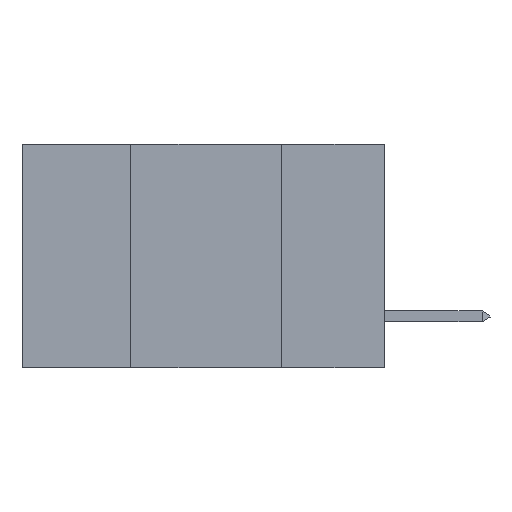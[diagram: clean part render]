
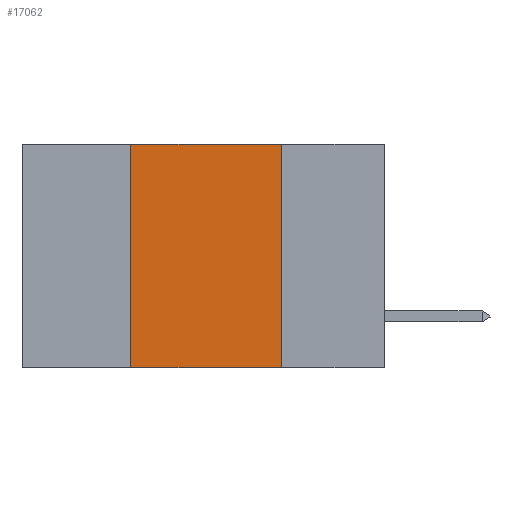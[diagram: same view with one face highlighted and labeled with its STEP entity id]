
A CAD part, left-side view. The second image highlights one B-rep face of the part: STEP entity #17062.
In plain terms, the highlighted planar face has unit normal (-1, 0, 0).
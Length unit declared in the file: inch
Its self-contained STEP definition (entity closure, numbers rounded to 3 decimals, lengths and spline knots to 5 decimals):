
#70 = VECTOR ( 'NONE', #6772, 39.37008 ) ;
#285 = FACE_OUTER_BOUND ( 'NONE', #20038, .T. ) ;
#735 = CARTESIAN_POINT ( 'NONE',  ( 0., 0.6, 0. ) ) ;
#895 = VERTEX_POINT ( 'NONE', #28042 ) ;
#1100 = CARTESIAN_POINT ( 'NONE',  ( 0., 0.17, -0.37 ) ) ;
#2730 = ORIENTED_EDGE ( 'NONE', *, *, #9376, .T. ) ;
#2997 = DIRECTION ( 'NONE',  ( 0., 0., -1. ) ) ;
#4866 = AXIS2_PLACEMENT_3D ( 'NONE', #735, #16094, #2997 ) ;
#5042 = EDGE_CURVE ( 'NONE', #6911, #27293, #19323, .T. ) ;
#5829 = LINE ( 'NONE', #23668, #70 ) ;
#6772 = DIRECTION ( 'NONE',  ( 0., 0., -1. ) ) ;
#6911 = VERTEX_POINT ( 'NONE', #19561 ) ;
#7093 = PLANE ( 'NONE',  #4866 ) ;
#7493 = LINE ( 'NONE', #16509, #17658 ) ;
#7668 = ORIENTED_EDGE ( 'NONE', *, *, #7778, .F. ) ;
#7778 = EDGE_CURVE ( 'NONE', #27293, #895, #23218, .T. ) ;
#8568 = VERTEX_POINT ( 'NONE', #1100 ) ;
#8936 = EDGE_CURVE ( 'NONE', #895, #8568, #5829, .T. ) ;
#9376 = EDGE_CURVE ( 'NONE', #6911, #8568, #7493, .T. ) ;
#14802 = CARTESIAN_POINT ( 'NONE',  ( 0., 0.6, 0. ) ) ;
#16094 = DIRECTION ( 'NONE',  ( 1., 0., 0. ) ) ;
#16509 = CARTESIAN_POINT ( 'NONE',  ( 0., 0.6, -0.37 ) ) ;
#17062 = ADVANCED_FACE ( 'NONE', ( #285 ), #7093, .F. ) ;
#17073 = DIRECTION ( 'NONE',  ( 0., -1., 0. ) ) ;
#17457 = VECTOR ( 'NONE', #17073, 39.37008 ) ;
#17658 = VECTOR ( 'NONE', #25060, 39.37008 ) ;
#18371 = ORIENTED_EDGE ( 'NONE', *, *, #5042, .F. ) ;
#19323 = LINE ( 'NONE', #21269, #21690 ) ;
#19561 = CARTESIAN_POINT ( 'NONE',  ( 0., 0.42, -0.37 ) ) ;
#20038 = EDGE_LOOP ( 'NONE', ( #24850, #7668, #18371, #2730 ) ) ;
#20682 = CARTESIAN_POINT ( 'NONE',  ( 0., 0.42, 0. ) ) ;
#21269 = CARTESIAN_POINT ( 'NONE',  ( 0., 0.42, 0. ) ) ;
#21690 = VECTOR ( 'NONE', #25822, 39.37008 ) ;
#23218 = LINE ( 'NONE', #14802, #17457 ) ;
#23668 = CARTESIAN_POINT ( 'NONE',  ( 0., 0.17, 0. ) ) ;
#24850 = ORIENTED_EDGE ( 'NONE', *, *, #8936, .F. ) ;
#25060 = DIRECTION ( 'NONE',  ( 0., -1., 0. ) ) ;
#25822 = DIRECTION ( 'NONE',  ( 0., 0., 1. ) ) ;
#27293 = VERTEX_POINT ( 'NONE', #20682 ) ;
#28042 = CARTESIAN_POINT ( 'NONE',  ( 0., 0.17, 0. ) ) ;
